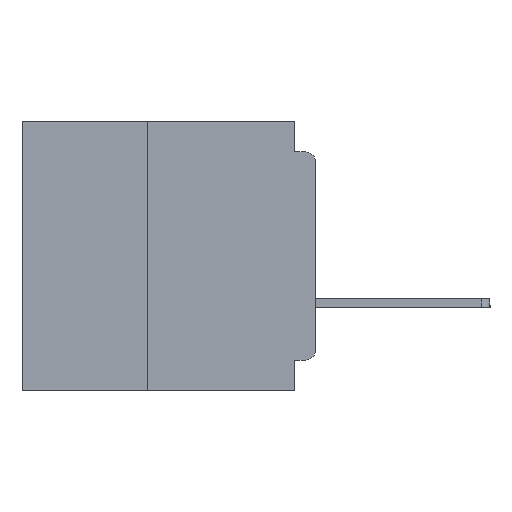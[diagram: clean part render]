
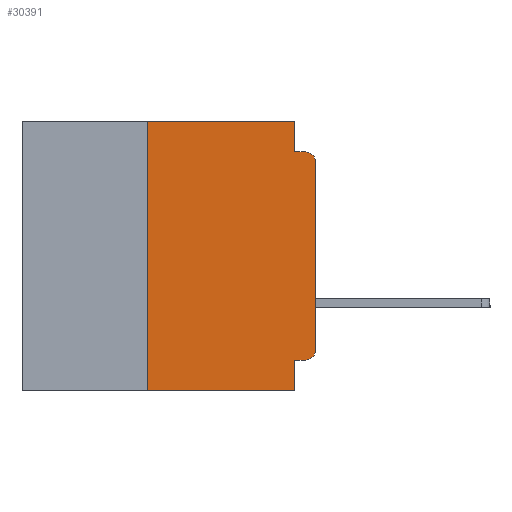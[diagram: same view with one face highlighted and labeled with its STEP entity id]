
A CAD part, left-side view. The second image highlights one B-rep face of the part: STEP entity #30391.
In plain terms, the highlighted planar face has unit normal (-1, 0, 0).
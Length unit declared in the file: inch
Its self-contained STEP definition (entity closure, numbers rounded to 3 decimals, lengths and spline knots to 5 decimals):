
#430 = EDGE_CURVE ( 'NONE', #57948, #45288, #41419, .T. ) ;
#788 = VERTEX_POINT ( 'NONE', #45745 ) ;
#2959 = CARTESIAN_POINT ( 'NONE',  ( 0., 0., 0. ) ) ;
#3123 = VECTOR ( 'NONE', #17961, 39.37008 ) ;
#3409 = VECTOR ( 'NONE', #7629, 39.37008 ) ;
#3898 = DIRECTION ( 'NONE',  ( 0., -1., 0. ) ) ;
#4421 = VERTEX_POINT ( 'NONE', #59690 ) ;
#4731 = AXIS2_PLACEMENT_3D ( 'NONE', #53202, #24989, #57929 ) ;
#7379 = PLANE ( 'NONE',  #39843 ) ;
#7550 = VECTOR ( 'NONE', #40963, 39.37008 ) ;
#7629 = DIRECTION ( 'NONE',  ( 0., 0., 1. ) ) ;
#10899 = EDGE_CURVE ( 'NONE', #58448, #4421, #15592, .T. ) ;
#11081 = CARTESIAN_POINT ( 'NONE',  ( 0., 0.031, -0.045 ) ) ;
#11940 = CARTESIAN_POINT ( 'NONE',  ( 0., 0.031, 0. ) ) ;
#12078 = CARTESIAN_POINT ( 'NONE',  ( 0., 0.437, 0. ) ) ;
#14179 = EDGE_CURVE ( 'NONE', #29031, #42495, #53577, .T. ) ;
#14996 = ORIENTED_EDGE ( 'NONE', *, *, #26436, .F. ) ;
#15592 = LINE ( 'NONE', #32246, #3123 ) ;
#16276 = VECTOR ( 'NONE', #28924, 39.37008 ) ;
#16958 = EDGE_CURVE ( 'NONE', #38906, #42495, #49570, .T. ) ;
#17961 = DIRECTION ( 'NONE',  ( 0., -1., 0. ) ) ;
#18617 = ORIENTED_EDGE ( 'NONE', *, *, #33669, .T. ) ;
#19053 = CARTESIAN_POINT ( 'NONE',  ( 0., 0.015, -0.06 ) ) ;
#20023 = ORIENTED_EDGE ( 'NONE', *, *, #14179, .T. ) ;
#20109 = LINE ( 'NONE', #59694, #7550 ) ;
#21796 = LINE ( 'NONE', #32175, #37349 ) ;
#21965 = EDGE_CURVE ( 'NONE', #58448, #54196, #20109, .T. ) ;
#23845 = DIRECTION ( 'NONE',  ( 0., 0., -1. ) ) ;
#24989 = DIRECTION ( 'NONE',  ( -1., 0., 0. ) ) ;
#26427 = DIRECTION ( 'NONE',  ( 1., 0., 0. ) ) ;
#26436 = EDGE_CURVE ( 'NONE', #54196, #60312, #21796, .T. ) ;
#27333 = ORIENTED_EDGE ( 'NONE', *, *, #21965, .F. ) ;
#27901 = AXIS2_PLACEMENT_3D ( 'NONE', #19053, #52089, #23845 ) ;
#28924 = DIRECTION ( 'NONE',  ( 0., 1., 0. ) ) ;
#29031 = VERTEX_POINT ( 'NONE', #44489 ) ;
#29881 = CARTESIAN_POINT ( 'NONE',  ( 0., 0., -0.045 ) ) ;
#30261 = CARTESIAN_POINT ( 'NONE',  ( 0., 0.031, -0.355 ) ) ;
#30391 = ADVANCED_FACE ( 'NONE', ( #53204 ), #7379, .F. ) ;
#31046 = DIRECTION ( 'NONE',  ( 0., 0., -1. ) ) ;
#32175 = CARTESIAN_POINT ( 'NONE',  ( 0., 0.437, 0. ) ) ;
#32246 = CARTESIAN_POINT ( 'NONE',  ( 0., 0.437, -0.4 ) ) ;
#33669 = EDGE_CURVE ( 'NONE', #788, #29031, #41050, .T. ) ;
#35606 = VECTOR ( 'NONE', #58261, 39.37008 ) ;
#35793 = CARTESIAN_POINT ( 'NONE',  ( 0., 0.25, 0. ) ) ;
#37349 = VECTOR ( 'NONE', #3898, 39.37008 ) ;
#38751 = ORIENTED_EDGE ( 'NONE', *, *, #40699, .T. ) ;
#38906 = VERTEX_POINT ( 'NONE', #11081 ) ;
#39843 = AXIS2_PLACEMENT_3D ( 'NONE', #12078, #26427, #59365 ) ;
#40699 = EDGE_CURVE ( 'NONE', #57948, #788, #60667, .T. ) ;
#40963 = DIRECTION ( 'NONE',  ( 0., 0., 1. ) ) ;
#41050 = LINE ( 'NONE', #2959, #3409 ) ;
#41419 = LINE ( 'NONE', #43122, #16276 ) ;
#41542 = CARTESIAN_POINT ( 'NONE',  ( 0., 0.015, -0.355 ) ) ;
#42495 = VERTEX_POINT ( 'NONE', #46561 ) ;
#43122 = CARTESIAN_POINT ( 'NONE',  ( 0., 0., -0.355 ) ) ;
#43222 = EDGE_LOOP ( 'NONE', ( #18617, #20023, #59754, #54337, #14996, #27333, #48537, #50503, #51184, #38751 ) ) ;
#44056 = DIRECTION ( 'NONE',  ( 0., 0., -1. ) ) ;
#44489 = CARTESIAN_POINT ( 'NONE',  ( 0., 0., -0.06 ) ) ;
#45288 = VERTEX_POINT ( 'NONE', #30261 ) ;
#45477 = VECTOR ( 'NONE', #31046, 39.37008 ) ;
#45745 = CARTESIAN_POINT ( 'NONE',  ( 0., 0., -0.34 ) ) ;
#45826 = CARTESIAN_POINT ( 'NONE',  ( 0., 0.25, -0.4 ) ) ;
#46561 = CARTESIAN_POINT ( 'NONE',  ( 0., 0.015, -0.045 ) ) ;
#48085 = EDGE_CURVE ( 'NONE', #45288, #4421, #50713, .T. ) ;
#48537 = ORIENTED_EDGE ( 'NONE', *, *, #10899, .T. ) ;
#48802 = EDGE_CURVE ( 'NONE', #60312, #38906, #57991, .T. ) ;
#49231 = VECTOR ( 'NONE', #44056, 39.37008 ) ;
#49570 = LINE ( 'NONE', #29881, #35606 ) ;
#50503 = ORIENTED_EDGE ( 'NONE', *, *, #48085, .F. ) ;
#50713 = LINE ( 'NONE', #58036, #49231 ) ;
#51184 = ORIENTED_EDGE ( 'NONE', *, *, #430, .F. ) ;
#52089 = DIRECTION ( 'NONE',  ( -1., 0., 0. ) ) ;
#53202 = CARTESIAN_POINT ( 'NONE',  ( 0., 0.015, -0.34 ) ) ;
#53204 = FACE_OUTER_BOUND ( 'NONE', #43222, .T. ) ;
#53577 = CIRCLE ( 'NONE', #27901, 0.015 ) ;
#54196 = VERTEX_POINT ( 'NONE', #35793 ) ;
#54337 = ORIENTED_EDGE ( 'NONE', *, *, #48802, .F. ) ;
#55668 = CARTESIAN_POINT ( 'NONE',  ( 0., 0.031, 0. ) ) ;
#57929 = DIRECTION ( 'NONE',  ( 0., 0., -1. ) ) ;
#57948 = VERTEX_POINT ( 'NONE', #41542 ) ;
#57991 = LINE ( 'NONE', #11940, #45477 ) ;
#58036 = CARTESIAN_POINT ( 'NONE',  ( 0., 0.031, -0.4 ) ) ;
#58261 = DIRECTION ( 'NONE',  ( 0., -1., 0. ) ) ;
#58448 = VERTEX_POINT ( 'NONE', #45826 ) ;
#59365 = DIRECTION ( 'NONE',  ( 0., 0., -1. ) ) ;
#59690 = CARTESIAN_POINT ( 'NONE',  ( 0., 0.031, -0.4 ) ) ;
#59694 = CARTESIAN_POINT ( 'NONE',  ( 0., 0.25, -0.4 ) ) ;
#59754 = ORIENTED_EDGE ( 'NONE', *, *, #16958, .F. ) ;
#60312 = VERTEX_POINT ( 'NONE', #55668 ) ;
#60667 = CIRCLE ( 'NONE', #4731, 0.015 ) ;
